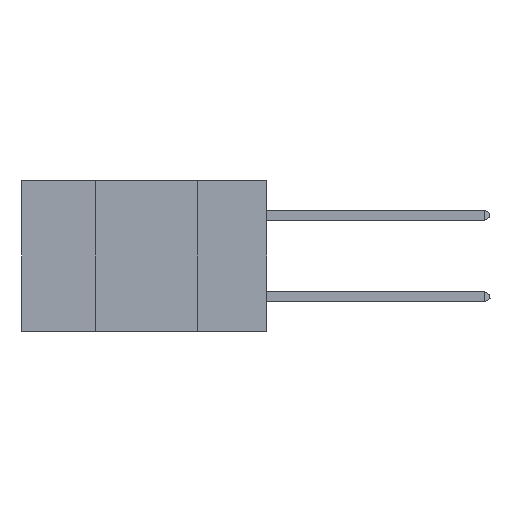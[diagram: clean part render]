
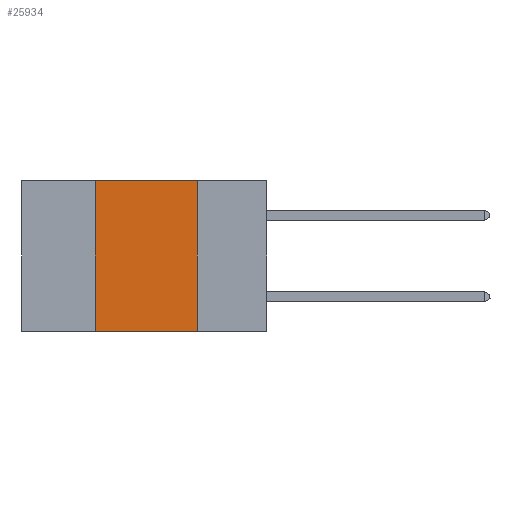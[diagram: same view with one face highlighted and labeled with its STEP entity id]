
A CAD part, left-side view. The second image highlights one B-rep face of the part: STEP entity #25934.
In plain terms, the highlighted planar face has unit normal (-1, 0, 0).
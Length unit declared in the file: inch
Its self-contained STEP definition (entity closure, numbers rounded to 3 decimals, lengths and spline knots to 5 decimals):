
#247 = EDGE_CURVE ( 'NONE', #29321, #10607, #22582, .T. ) ;
#1889 = DIRECTION ( 'NONE',  ( 0., -1., 0. ) ) ;
#2430 = FACE_OUTER_BOUND ( 'NONE', #4630, .T. ) ;
#3747 = ORIENTED_EDGE ( 'NONE', *, *, #32804, .F. ) ;
#3951 = VECTOR ( 'NONE', #7848, 39.37008 ) ;
#4630 = EDGE_LOOP ( 'NONE', ( #36169, #3747, #21839, #18683 ) ) ;
#7184 = CARTESIAN_POINT ( 'NONE',  ( 0., 0.42, -0.37 ) ) ;
#7848 = DIRECTION ( 'NONE',  ( 0., 0., 1. ) ) ;
#9214 = CARTESIAN_POINT ( 'NONE',  ( 0., 0.6, 0. ) ) ;
#10607 = VERTEX_POINT ( 'NONE', #23500 ) ;
#11040 = DIRECTION ( 'NONE',  ( 0., 0., -1. ) ) ;
#13771 = EDGE_CURVE ( 'NONE', #21447, #15313, #20625, .T. ) ;
#14074 = CARTESIAN_POINT ( 'NONE',  ( 0., 0.6, -0.37 ) ) ;
#14212 = DIRECTION ( 'NONE',  ( 0., -1., 0. ) ) ;
#14279 = LINE ( 'NONE', #35046, #29139 ) ;
#15313 = VERTEX_POINT ( 'NONE', #20966 ) ;
#15766 = VECTOR ( 'NONE', #14212, 39.37008 ) ;
#16659 = CARTESIAN_POINT ( 'NONE',  ( 0., 0.42, 0. ) ) ;
#18040 = PLANE ( 'NONE',  #30337 ) ;
#18432 = DIRECTION ( 'NONE',  ( 0., 0., -1. ) ) ;
#18683 = ORIENTED_EDGE ( 'NONE', *, *, #27343, .T. ) ;
#20625 = LINE ( 'NONE', #16659, #3951 ) ;
#20966 = CARTESIAN_POINT ( 'NONE',  ( 0., 0.42, 0. ) ) ;
#21447 = VERTEX_POINT ( 'NONE', #7184 ) ;
#21839 = ORIENTED_EDGE ( 'NONE', *, *, #13771, .F. ) ;
#22582 = LINE ( 'NONE', #29760, #38395 ) ;
#23500 = CARTESIAN_POINT ( 'NONE',  ( 0., 0.17, -0.37 ) ) ;
#23883 = LINE ( 'NONE', #14074, #15766 ) ;
#25934 = ADVANCED_FACE ( 'NONE', ( #2430 ), #18040, .F. ) ;
#27252 = CARTESIAN_POINT ( 'NONE',  ( 0., 0.17, 0. ) ) ;
#27343 = EDGE_CURVE ( 'NONE', #21447, #10607, #23883, .T. ) ;
#29139 = VECTOR ( 'NONE', #1889, 39.37008 ) ;
#29321 = VERTEX_POINT ( 'NONE', #27252 ) ;
#29760 = CARTESIAN_POINT ( 'NONE',  ( 0., 0.17, 0. ) ) ;
#30337 = AXIS2_PLACEMENT_3D ( 'NONE', #9214, #34227, #18432 ) ;
#32804 = EDGE_CURVE ( 'NONE', #15313, #29321, #14279, .T. ) ;
#34227 = DIRECTION ( 'NONE',  ( 1., 0., 0. ) ) ;
#35046 = CARTESIAN_POINT ( 'NONE',  ( 0., 0.6, 0. ) ) ;
#36169 = ORIENTED_EDGE ( 'NONE', *, *, #247, .F. ) ;
#38395 = VECTOR ( 'NONE', #11040, 39.37008 ) ;
